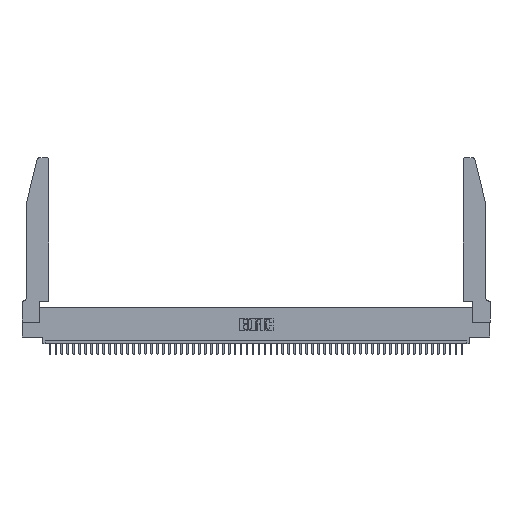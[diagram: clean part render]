
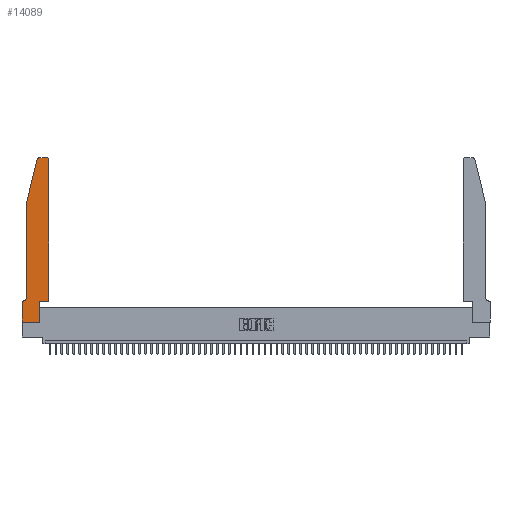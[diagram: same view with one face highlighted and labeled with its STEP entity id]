
A CAD part, top view. The second image highlights one B-rep face of the part: STEP entity #14089.
In plain terms, the highlighted planar face has unit normal (0, 0, 1).
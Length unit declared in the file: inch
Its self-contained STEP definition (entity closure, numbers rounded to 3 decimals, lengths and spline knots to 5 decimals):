
#25 = CARTESIAN_POINT ( 'NONE',  ( 0.2605, 2.75, 0.37 ) ) ;
#371 = VERTEX_POINT ( 'NONE', #865 ) ;
#865 = CARTESIAN_POINT ( 'NONE',  ( 0.2865, 0.35, 0.37 ) ) ;
#1115 = EDGE_LOOP ( 'NONE', ( #15728, #23815, #7105, #14006, #41903, #9217, #14955, #12377, #32459, #41096, #42185, #14408 ) ) ;
#1492 = DIRECTION ( 'NONE',  ( 0., 1., 0. ) ) ;
#2497 = VECTOR ( 'NONE', #8490, 39.37008 ) ;
#2961 = DIRECTION ( 'NONE',  ( -0.239, -0.971, 0. ) ) ;
#3698 = CIRCLE ( 'NONE', #6324, 0.03 ) ;
#4313 = CARTESIAN_POINT ( 'NONE',  ( 0., 0., 0.37 ) ) ;
#4665 = CARTESIAN_POINT ( 'NONE',  ( 0.2865, 0.35, 0.37 ) ) ;
#4840 = AXIS2_PLACEMENT_3D ( 'NONE', #18346, #39294, #13968 ) ;
#5611 = VECTOR ( 'NONE', #42615, 39.37008 ) ;
#5730 = VERTEX_POINT ( 'NONE', #44602 ) ;
#6266 = VECTOR ( 'NONE', #23627, 39.37008 ) ;
#6324 = AXIS2_PLACEMENT_3D ( 'NONE', #50476, #12461, #50302 ) ;
#7105 = ORIENTED_EDGE ( 'NONE', *, *, #43252, .T. ) ;
#7126 = CARTESIAN_POINT ( 'NONE',  ( 0.4505, 0.35, 0.37 ) ) ;
#7182 = EDGE_CURVE ( 'NONE', #5730, #40644, #3698, .T. ) ;
#7512 = CARTESIAN_POINT ( 'NONE',  ( 0.0755, 2., 0.37 ) ) ;
#7742 = EDGE_CURVE ( 'NONE', #9827, #47784, #10033, .T. ) ;
#7856 = CARTESIAN_POINT ( 'NONE',  ( 0.4205, 2.72, 0.37 ) ) ;
#8353 = CARTESIAN_POINT ( 'NONE',  ( 0.0055, 0.42, 0.37 ) ) ;
#8490 = DIRECTION ( 'NONE',  ( -1., 0., 0. ) ) ;
#8606 = VECTOR ( 'NONE', #37888, 39.37008 ) ;
#9058 = VERTEX_POINT ( 'NONE', #17339 ) ;
#9217 = ORIENTED_EDGE ( 'NONE', *, *, #22972, .T. ) ;
#9827 = VERTEX_POINT ( 'NONE', #23969 ) ;
#9839 = EDGE_CURVE ( 'NONE', #13395, #41832, #53451, .T. ) ;
#10033 = LINE ( 'NONE', #7126, #47171 ) ;
#10815 = VERTEX_POINT ( 'NONE', #29675 ) ;
#12344 = CARTESIAN_POINT ( 'NONE',  ( 0.4205, 2.75, 0.37 ) ) ;
#12377 = ORIENTED_EDGE ( 'NONE', *, *, #41388, .T. ) ;
#12461 = DIRECTION ( 'NONE',  ( 0., 0., 1. ) ) ;
#12783 = EDGE_CURVE ( 'NONE', #42768, #371, #18556, .T. ) ;
#13030 = CARTESIAN_POINT ( 'NONE',  ( 0.0755, 2., 0.37 ) ) ;
#13395 = VERTEX_POINT ( 'NONE', #13030 ) ;
#13968 = DIRECTION ( 'NONE',  ( 1., 0., 0. ) ) ;
#14006 = ORIENTED_EDGE ( 'NONE', *, *, #9839, .T. ) ;
#14089 = ADVANCED_FACE ( 'NONE', ( #29423 ), #43503, .T. ) ;
#14408 = ORIENTED_EDGE ( 'NONE', *, *, #25455, .T. ) ;
#14955 = ORIENTED_EDGE ( 'NONE', *, *, #17864, .T. ) ;
#15683 = AXIS2_PLACEMENT_3D ( 'NONE', #8353, #24657, #46333 ) ;
#15728 = ORIENTED_EDGE ( 'NONE', *, *, #16933, .T. ) ;
#16906 = CIRCLE ( 'NONE', #52204, 0.03 ) ;
#16933 = EDGE_CURVE ( 'NONE', #41715, #5730, #31806, .T. ) ;
#17339 = CARTESIAN_POINT ( 'NONE',  ( 0., 0., 0.37 ) ) ;
#17864 = EDGE_CURVE ( 'NONE', #10815, #9058, #32300, .T. ) ;
#18253 = LINE ( 'NONE', #23942, #26698 ) ;
#18346 = CARTESIAN_POINT ( 'NONE',  ( 0., 0.35, 0.37 ) ) ;
#18556 = LINE ( 'NONE', #4665, #5611 ) ;
#18722 = CARTESIAN_POINT ( 'NONE',  ( 0., 0., 0.37 ) ) ;
#20914 = LINE ( 'NONE', #4313, #8606 ) ;
#22972 = EDGE_CURVE ( 'NONE', #48675, #10815, #30387, .T. ) ;
#23627 = DIRECTION ( 'NONE',  ( 0., -1., 0. ) ) ;
#23815 = ORIENTED_EDGE ( 'NONE', *, *, #7182, .T. ) ;
#23942 = CARTESIAN_POINT ( 'NONE',  ( 0.4505, 0.35, 0.37 ) ) ;
#23969 = CARTESIAN_POINT ( 'NONE',  ( 0.4505, 0.35, 0.37 ) ) ;
#24513 = DIRECTION ( 'NONE',  ( 0., 0., 1. ) ) ;
#24657 = DIRECTION ( 'NONE',  ( 0., 0., -1. ) ) ;
#25455 = EDGE_CURVE ( 'NONE', #47784, #41715, #16906, .T. ) ;
#26698 = VECTOR ( 'NONE', #36159, 39.37008 ) ;
#28981 = EDGE_CURVE ( 'NONE', #41832, #48675, #46452, .T. ) ;
#29423 = FACE_OUTER_BOUND ( 'NONE', #1115, .T. ) ;
#29591 = LINE ( 'NONE', #44751, #44617 ) ;
#29675 = CARTESIAN_POINT ( 'NONE',  ( 0., 0.35, 0.37 ) ) ;
#30387 = LINE ( 'NONE', #40944, #2497 ) ;
#31154 = VECTOR ( 'NONE', #32759, 39.37008 ) ;
#31806 = LINE ( 'NONE', #25, #31154 ) ;
#32300 = LINE ( 'NONE', #18722, #6266 ) ;
#32459 = ORIENTED_EDGE ( 'NONE', *, *, #12783, .T. ) ;
#32630 = CARTESIAN_POINT ( 'NONE',  ( 0.2865, 0., 0.37 ) ) ;
#32759 = DIRECTION ( 'NONE',  ( -1., 0., 0. ) ) ;
#34497 = VECTOR ( 'NONE', #36550, 39.37008 ) ;
#35437 = DIRECTION ( 'NONE',  ( 1., 0., 0. ) ) ;
#36159 = DIRECTION ( 'NONE',  ( 1., 0., 0. ) ) ;
#36550 = DIRECTION ( 'NONE',  ( 0., -1., 0. ) ) ;
#37888 = DIRECTION ( 'NONE',  ( 1., 0., 0. ) ) ;
#38685 = CARTESIAN_POINT ( 'NONE',  ( 0.0055, 0.35, 0.37 ) ) ;
#39294 = DIRECTION ( 'NONE',  ( 0., 0., 1. ) ) ;
#40644 = VERTEX_POINT ( 'NONE', #48191 ) ;
#40944 = CARTESIAN_POINT ( 'NONE',  ( 0.0755, 0.35, 0.37 ) ) ;
#41096 = ORIENTED_EDGE ( 'NONE', *, *, #45478, .T. ) ;
#41388 = EDGE_CURVE ( 'NONE', #9058, #42768, #20914, .T. ) ;
#41715 = VERTEX_POINT ( 'NONE', #12344 ) ;
#41832 = VERTEX_POINT ( 'NONE', #46528 ) ;
#41903 = ORIENTED_EDGE ( 'NONE', *, *, #28981, .T. ) ;
#42185 = ORIENTED_EDGE ( 'NONE', *, *, #7742, .T. ) ;
#42615 = DIRECTION ( 'NONE',  ( 0., 1., 0. ) ) ;
#42768 = VERTEX_POINT ( 'NONE', #32630 ) ;
#43252 = EDGE_CURVE ( 'NONE', #40644, #13395, #29591, .T. ) ;
#43503 = PLANE ( 'NONE',  #4840 ) ;
#44602 = CARTESIAN_POINT ( 'NONE',  ( 0.284, 2.75, 0.37 ) ) ;
#44617 = VECTOR ( 'NONE', #2961, 39.37008 ) ;
#44751 = CARTESIAN_POINT ( 'NONE',  ( 0.0755, 2., 0.37 ) ) ;
#45478 = EDGE_CURVE ( 'NONE', #371, #9827, #18253, .T. ) ;
#46333 = DIRECTION ( 'NONE',  ( -1., 0., 0. ) ) ;
#46452 = CIRCLE ( 'NONE', #15683, 0.07 ) ;
#46528 = CARTESIAN_POINT ( 'NONE',  ( 0.0755, 0.42, 0.37 ) ) ;
#47171 = VECTOR ( 'NONE', #1492, 39.37008 ) ;
#47784 = VERTEX_POINT ( 'NONE', #49029 ) ;
#48191 = CARTESIAN_POINT ( 'NONE',  ( 0.25487, 2.72718, 0.37 ) ) ;
#48675 = VERTEX_POINT ( 'NONE', #38685 ) ;
#49029 = CARTESIAN_POINT ( 'NONE',  ( 0.4505, 2.72, 0.37 ) ) ;
#50302 = DIRECTION ( 'NONE',  ( 1., 0., 0. ) ) ;
#50476 = CARTESIAN_POINT ( 'NONE',  ( 0.284, 2.72, 0.37 ) ) ;
#52204 = AXIS2_PLACEMENT_3D ( 'NONE', #7856, #24513, #35437 ) ;
#53451 = LINE ( 'NONE', #7512, #34497 ) ;
